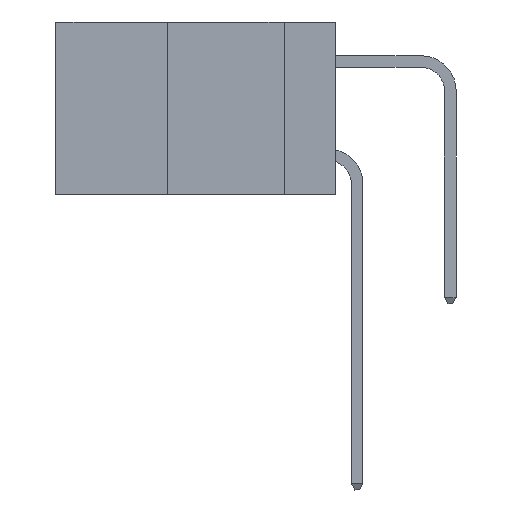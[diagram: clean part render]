
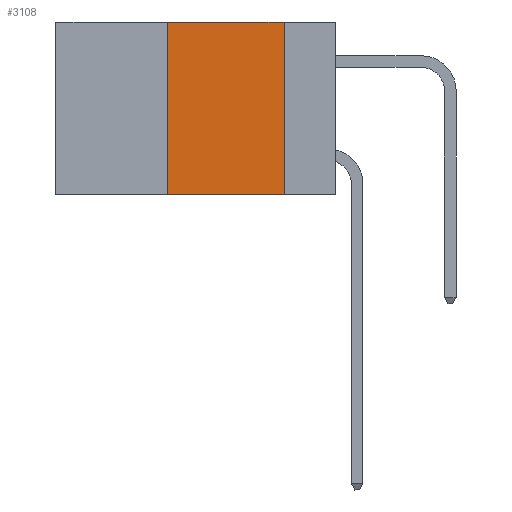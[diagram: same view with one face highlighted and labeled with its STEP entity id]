
A CAD part, left-side view. The second image highlights one B-rep face of the part: STEP entity #3108.
In plain terms, the highlighted planar face has unit normal (-1, 0, 0).
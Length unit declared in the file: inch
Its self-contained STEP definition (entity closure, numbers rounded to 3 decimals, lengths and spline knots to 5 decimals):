
#245 = VERTEX_POINT ( 'NONE', #16199 ) ;
#494 = EDGE_CURVE ( 'NONE', #8577, #14590, #18039, .T. ) ;
#570 = LINE ( 'NONE', #815, #17432 ) ;
#815 = CARTESIAN_POINT ( 'NONE',  ( 0., 0.36, 0. ) ) ;
#1581 = LINE ( 'NONE', #6912, #7002 ) ;
#1684 = EDGE_LOOP ( 'NONE', ( #11807, #16577, #4066, #12818 ) ) ;
#3108 = ADVANCED_FACE ( 'NONE', ( #6005 ), #13211, .F. ) ;
#3225 = LINE ( 'NONE', #7359, #15761 ) ;
#3354 = DIRECTION ( 'NONE',  ( 1., 0., 0. ) ) ;
#4066 = ORIENTED_EDGE ( 'NONE', *, *, #8017, .F. ) ;
#4812 = VERTEX_POINT ( 'NONE', #12238 ) ;
#6005 = FACE_OUTER_BOUND ( 'NONE', #1684, .T. ) ;
#6788 = DIRECTION ( 'NONE',  ( 0., -1., 0. ) ) ;
#6912 = CARTESIAN_POINT ( 'NONE',  ( 0., 0.11, 0. ) ) ;
#7002 = VECTOR ( 'NONE', #18223, 39.37008 ) ;
#7359 = CARTESIAN_POINT ( 'NONE',  ( 0., 0.6, -0.37 ) ) ;
#8017 = EDGE_CURVE ( 'NONE', #4812, #8577, #570, .T. ) ;
#8275 = CARTESIAN_POINT ( 'NONE',  ( 0., 0.6, 0. ) ) ;
#8577 = VERTEX_POINT ( 'NONE', #20111 ) ;
#9144 = EDGE_CURVE ( 'NONE', #14590, #245, #1581, .T. ) ;
#11807 = ORIENTED_EDGE ( 'NONE', *, *, #9144, .F. ) ;
#12238 = CARTESIAN_POINT ( 'NONE',  ( 0., 0.36, -0.37 ) ) ;
#12818 = ORIENTED_EDGE ( 'NONE', *, *, #19222, .T. ) ;
#13211 = PLANE ( 'NONE',  #16843 ) ;
#13825 = VECTOR ( 'NONE', #6788, 39.37008 ) ;
#14590 = VERTEX_POINT ( 'NONE', #17490 ) ;
#14805 = DIRECTION ( 'NONE',  ( 0., 0., -1. ) ) ;
#15761 = VECTOR ( 'NONE', #17161, 39.37008 ) ;
#16199 = CARTESIAN_POINT ( 'NONE',  ( 0., 0.11, -0.37 ) ) ;
#16577 = ORIENTED_EDGE ( 'NONE', *, *, #494, .F. ) ;
#16843 = AXIS2_PLACEMENT_3D ( 'NONE', #8275, #3354, #14805 ) ;
#17161 = DIRECTION ( 'NONE',  ( 0., -1., 0. ) ) ;
#17432 = VECTOR ( 'NONE', #20280, 39.37008 ) ;
#17490 = CARTESIAN_POINT ( 'NONE',  ( 0., 0.11, 0. ) ) ;
#18039 = LINE ( 'NONE', #20806, #13825 ) ;
#18223 = DIRECTION ( 'NONE',  ( 0., 0., -1. ) ) ;
#19222 = EDGE_CURVE ( 'NONE', #4812, #245, #3225, .T. ) ;
#20111 = CARTESIAN_POINT ( 'NONE',  ( 0., 0.36, 0. ) ) ;
#20280 = DIRECTION ( 'NONE',  ( 0., 0., 1. ) ) ;
#20806 = CARTESIAN_POINT ( 'NONE',  ( 0., 0.6, 0. ) ) ;
